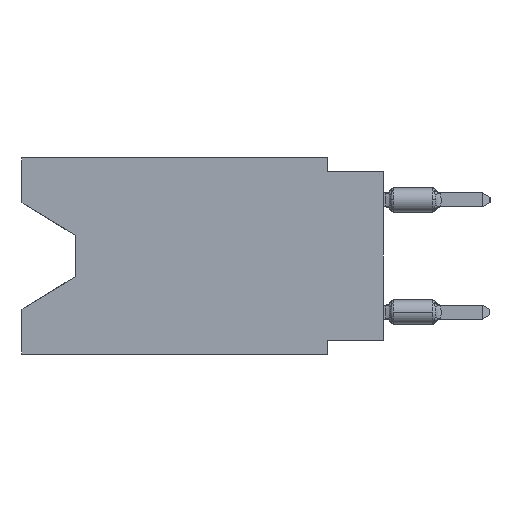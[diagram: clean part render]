
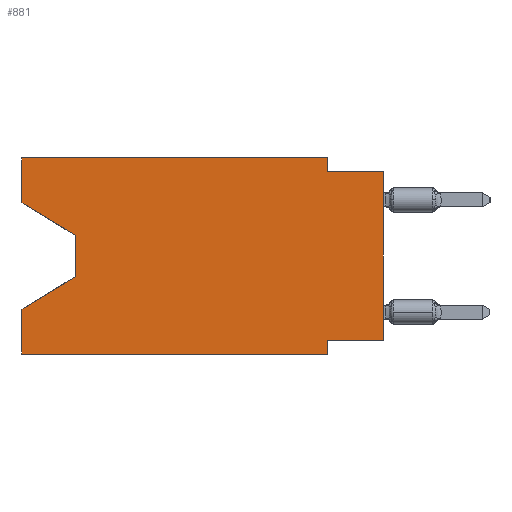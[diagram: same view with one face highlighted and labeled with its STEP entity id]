
A CAD part, left-side view. The second image highlights one B-rep face of the part: STEP entity #881.
In plain terms, the highlighted planar face has unit normal (-1, 0, 0).
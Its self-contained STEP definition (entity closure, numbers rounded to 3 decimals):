
#47 = ORIENTED_EDGE ( 'NONE', *, *, #16149, .T. ) ;
#289 = CARTESIAN_POINT ( 'NONE',  ( 0., 0., -8.255 ) ) ;
#680 = VERTEX_POINT ( 'NONE', #12369 ) ;
#881 = ADVANCED_FACE ( 'NONE', ( #1308 ), #29552, .F. ) ;
#946 = DIRECTION ( 'NONE',  ( 0., -1., 0. ) ) ;
#1308 = FACE_OUTER_BOUND ( 'NONE', #16353, .T. ) ;
#1760 = ORIENTED_EDGE ( 'NONE', *, *, #26781, .F. ) ;
#3405 = LINE ( 'NONE', #26819, #18342 ) ;
#3622 = EDGE_CURVE ( 'NONE', #15669, #24314, #26505, .T. ) ;
#3750 = ORIENTED_EDGE ( 'NONE', *, *, #21912, .F. ) ;
#4003 = DIRECTION ( 'NONE',  ( 0., 0., 1. ) ) ;
#4059 = CARTESIAN_POINT ( 'NONE',  ( 0., 2.54, -8.89 ) ) ;
#4116 = CARTESIAN_POINT ( 'NONE',  ( 0., 16.383, 0. ) ) ;
#4127 = EDGE_CURVE ( 'NONE', #24314, #26295, #3405, .T. ) ;
#4754 = VECTOR ( 'NONE', #12839, 1000. ) ;
#4819 = DIRECTION ( 'NONE',  ( 0., 1., 0. ) ) ;
#5182 = VECTOR ( 'NONE', #9077, 1000. ) ;
#5215 = VERTEX_POINT ( 'NONE', #16834 ) ;
#5443 = CARTESIAN_POINT ( 'NONE',  ( 0., 16.383, 0. ) ) ;
#5821 = ORIENTED_EDGE ( 'NONE', *, *, #3622, .F. ) ;
#6596 = VERTEX_POINT ( 'NONE', #12606 ) ;
#6898 = CARTESIAN_POINT ( 'NONE',  ( 0., 13.97, -3.505 ) ) ;
#7144 = EDGE_CURVE ( 'NONE', #680, #17982, #30383, .T. ) ;
#8244 = VECTOR ( 'NONE', #21869, 1000. ) ;
#8379 = DIRECTION ( 'NONE',  ( 0., -1., 0. ) ) ;
#8620 = DIRECTION ( 'NONE',  ( 0., 0., -1. ) ) ;
#9077 = DIRECTION ( 'NONE',  ( 0., 0., -1. ) ) ;
#9159 = LINE ( 'NONE', #20879, #25064 ) ;
#9330 = VERTEX_POINT ( 'NONE', #25506 ) ;
#9409 = LINE ( 'NONE', #9551, #8244 ) ;
#9551 = CARTESIAN_POINT ( 'NONE',  ( 0., 16.383, 0. ) ) ;
#9909 = VECTOR ( 'NONE', #30100, 1000. ) ;
#10089 = LINE ( 'NONE', #289, #16233 ) ;
#10090 = VERTEX_POINT ( 'NONE', #4059 ) ;
#10551 = VERTEX_POINT ( 'NONE', #22888 ) ;
#10659 = VECTOR ( 'NONE', #18681, 1000. ) ;
#11025 = ORIENTED_EDGE ( 'NONE', *, *, #25710, .T. ) ;
#11655 = ORIENTED_EDGE ( 'NONE', *, *, #17225, .F. ) ;
#11718 = CARTESIAN_POINT ( 'NONE',  ( 0., 2.54, -8.89 ) ) ;
#12212 = EDGE_CURVE ( 'NONE', #15201, #10090, #14005, .T. ) ;
#12289 = DIRECTION ( 'NONE',  ( 0., 0., 1. ) ) ;
#12293 = ORIENTED_EDGE ( 'NONE', *, *, #4127, .F. ) ;
#12369 = CARTESIAN_POINT ( 'NONE',  ( 0., 0., -8.255 ) ) ;
#12606 = CARTESIAN_POINT ( 'NONE',  ( 0., 2.54, -8.255 ) ) ;
#12780 = LINE ( 'NONE', #14970, #21868 ) ;
#12839 = DIRECTION ( 'NONE',  ( 0., -0.855, -0.519 ) ) ;
#13709 = CARTESIAN_POINT ( 'NONE',  ( 0., 13.97, -5.385 ) ) ;
#14005 = LINE ( 'NONE', #25562, #10659 ) ;
#14837 = ORIENTED_EDGE ( 'NONE', *, *, #12212, .T. ) ;
#14970 = CARTESIAN_POINT ( 'NONE',  ( 0., 0., -0.635 ) ) ;
#15201 = VERTEX_POINT ( 'NONE', #19737 ) ;
#15669 = VERTEX_POINT ( 'NONE', #20000 ) ;
#16002 = VECTOR ( 'NONE', #27746, 1000. ) ;
#16149 = EDGE_CURVE ( 'NONE', #10551, #5215, #25434, .T. ) ;
#16233 = VECTOR ( 'NONE', #4819, 1000. ) ;
#16353 = EDGE_LOOP ( 'NONE', ( #28673, #11025, #47, #1760, #14837, #3750, #22049, #22660, #11655, #25430, #12293, #5821 ) ) ;
#16834 = CARTESIAN_POINT ( 'NONE',  ( 0., 16.383, -6.852 ) ) ;
#17225 = EDGE_CURVE ( 'NONE', #9330, #17982, #12780, .T. ) ;
#17982 = VERTEX_POINT ( 'NONE', #23811 ) ;
#18110 = VECTOR ( 'NONE', #12289, 1000. ) ;
#18342 = VECTOR ( 'NONE', #8379, 1000. ) ;
#18495 = CARTESIAN_POINT ( 'NONE',  ( 0., 0., 0. ) ) ;
#18675 = DIRECTION ( 'NONE',  ( 0., 0., -1. ) ) ;
#18681 = DIRECTION ( 'NONE',  ( 0., -1., 0. ) ) ;
#19737 = CARTESIAN_POINT ( 'NONE',  ( 0., 16.383, -8.89 ) ) ;
#20000 = CARTESIAN_POINT ( 'NONE',  ( 0., 16.383, -2.038 ) ) ;
#20769 = EDGE_CURVE ( 'NONE', #680, #6596, #10089, .T. ) ;
#20879 = CARTESIAN_POINT ( 'NONE',  ( 0., 2.54, 0. ) ) ;
#21868 = VECTOR ( 'NONE', #946, 1000. ) ;
#21869 = DIRECTION ( 'NONE',  ( 0., 0., 1. ) ) ;
#21912 = EDGE_CURVE ( 'NONE', #6596, #10090, #25940, .T. ) ;
#22049 = ORIENTED_EDGE ( 'NONE', *, *, #20769, .F. ) ;
#22300 = AXIS2_PLACEMENT_3D ( 'NONE', #4116, #25179, #8620 ) ;
#22660 = ORIENTED_EDGE ( 'NONE', *, *, #7144, .T. ) ;
#22824 = CARTESIAN_POINT ( 'NONE',  ( 0., 16.383, -2.038 ) ) ;
#22888 = CARTESIAN_POINT ( 'NONE',  ( 0., 13.97, -5.385 ) ) ;
#23739 = VERTEX_POINT ( 'NONE', #6898 ) ;
#23811 = CARTESIAN_POINT ( 'NONE',  ( 0., 0., -0.635 ) ) ;
#24153 = CARTESIAN_POINT ( 'NONE',  ( 0., 16.383, 0. ) ) ;
#24314 = VERTEX_POINT ( 'NONE', #5443 ) ;
#24562 = EDGE_CURVE ( 'NONE', #26295, #9330, #9159, .T. ) ;
#24893 = VECTOR ( 'NONE', #4003, 1000. ) ;
#25064 = VECTOR ( 'NONE', #18675, 1000. ) ;
#25089 = LINE ( 'NONE', #27577, #16002 ) ;
#25179 = DIRECTION ( 'NONE',  ( 1., 0., 0. ) ) ;
#25430 = ORIENTED_EDGE ( 'NONE', *, *, #24562, .F. ) ;
#25434 = LINE ( 'NONE', #13709, #9909 ) ;
#25506 = CARTESIAN_POINT ( 'NONE',  ( 0., 2.54, -0.635 ) ) ;
#25562 = CARTESIAN_POINT ( 'NONE',  ( 0., 16.383, -8.89 ) ) ;
#25710 = EDGE_CURVE ( 'NONE', #23739, #10551, #25089, .T. ) ;
#25940 = LINE ( 'NONE', #11718, #5182 ) ;
#25988 = CARTESIAN_POINT ( 'NONE',  ( 0., 2.54, 0. ) ) ;
#26295 = VERTEX_POINT ( 'NONE', #25988 ) ;
#26505 = LINE ( 'NONE', #24153, #18110 ) ;
#26568 = EDGE_CURVE ( 'NONE', #15669, #23739, #29544, .T. ) ;
#26781 = EDGE_CURVE ( 'NONE', #15201, #5215, #9409, .T. ) ;
#26819 = CARTESIAN_POINT ( 'NONE',  ( 0., 16.383, 0. ) ) ;
#27577 = CARTESIAN_POINT ( 'NONE',  ( 0., 13.97, -3.505 ) ) ;
#27746 = DIRECTION ( 'NONE',  ( 0., 0., -1. ) ) ;
#28673 = ORIENTED_EDGE ( 'NONE', *, *, #26568, .T. ) ;
#29544 = LINE ( 'NONE', #22824, #4754 ) ;
#29552 = PLANE ( 'NONE',  #22300 ) ;
#30100 = DIRECTION ( 'NONE',  ( 0., 0.855, -0.519 ) ) ;
#30383 = LINE ( 'NONE', #18495, #24893 ) ;
